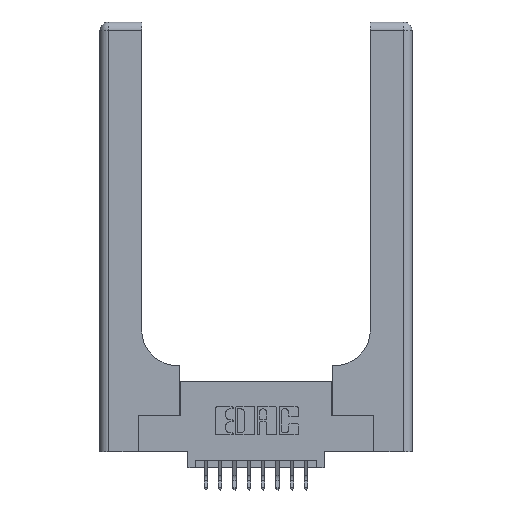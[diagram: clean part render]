
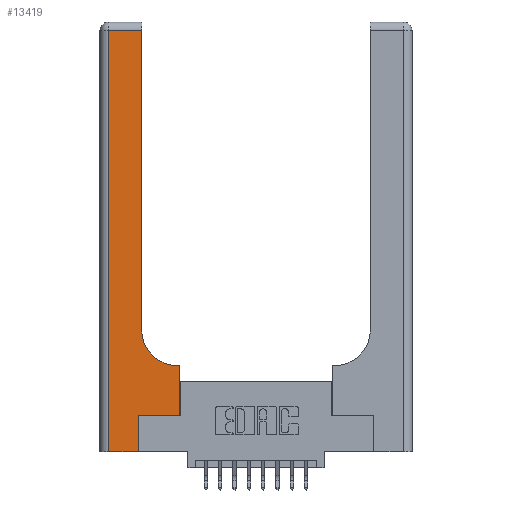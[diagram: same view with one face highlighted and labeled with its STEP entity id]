
A CAD part, top view. The second image highlights one B-rep face of the part: STEP entity #13419.
In plain terms, the highlighted planar face has unit normal (0, 0, 1).
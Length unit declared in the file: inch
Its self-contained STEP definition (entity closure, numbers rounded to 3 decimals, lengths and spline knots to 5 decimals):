
#223 = ORIENTED_EDGE ( 'NONE', *, *, #3497, .T. ) ;
#546 = CARTESIAN_POINT ( 'NONE',  ( 0., 0., 0.37 ) ) ;
#769 = CARTESIAN_POINT ( 'NONE',  ( 0.5585, 0.25, 0.37 ) ) ;
#796 = LINE ( 'NONE', #11181, #9317 ) ;
#807 = CARTESIAN_POINT ( 'NONE',  ( 0., 3., 0.37 ) ) ;
#1015 = EDGE_CURVE ( 'NONE', #10099, #3029, #2686, .T. ) ;
#1097 = VECTOR ( 'NONE', #10924, 39.37008 ) ;
#1381 = FACE_OUTER_BOUND ( 'NONE', #1650, .T. ) ;
#1394 = LINE ( 'NONE', #5864, #2605 ) ;
#1650 = EDGE_LOOP ( 'NONE', ( #8030, #5851, #15524, #223, #15790, #3409, #6822, #12961, #12147 ) ) ;
#1975 = DIRECTION ( 'NONE',  ( 1., 0., 0. ) ) ;
#1995 = VECTOR ( 'NONE', #3633, 39.37008 ) ;
#2091 = DIRECTION ( 'NONE',  ( -1., 0., 0. ) ) ;
#2115 = CARTESIAN_POINT ( 'NONE',  ( 0.269, 0., 0.37 ) ) ;
#2591 = CARTESIAN_POINT ( 'NONE',  ( 0.5415, 0.6, 0.37 ) ) ;
#2605 = VECTOR ( 'NONE', #5752, 39.37008 ) ;
#2686 = CIRCLE ( 'NONE', #16334, 0.25 ) ;
#3011 = CARTESIAN_POINT ( 'NONE',  ( 0.2915, 2.94, 0.37 ) ) ;
#3029 = VERTEX_POINT ( 'NONE', #15303 ) ;
#3409 = ORIENTED_EDGE ( 'NONE', *, *, #9844, .T. ) ;
#3497 = EDGE_CURVE ( 'NONE', #9450, #12011, #4415, .T. ) ;
#3633 = DIRECTION ( 'NONE',  ( 1., 0., 0. ) ) ;
#3676 = CARTESIAN_POINT ( 'NONE',  ( 0.06, 0., 0.37 ) ) ;
#4402 = DIRECTION ( 'NONE',  ( 0., 1., 0. ) ) ;
#4415 = LINE ( 'NONE', #546, #7609 ) ;
#4424 = EDGE_CURVE ( 'NONE', #12011, #5000, #15259, .T. ) ;
#4976 = EDGE_CURVE ( 'NONE', #3029, #5951, #13787, .T. ) ;
#5000 = VERTEX_POINT ( 'NONE', #8362 ) ;
#5591 = AXIS2_PLACEMENT_3D ( 'NONE', #807, #8357, #2091 ) ;
#5752 = DIRECTION ( 'NONE',  ( 0., -1., 0. ) ) ;
#5843 = DIRECTION ( 'NONE',  ( 0., 1., 0. ) ) ;
#5851 = ORIENTED_EDGE ( 'NONE', *, *, #7444, .T. ) ;
#5860 = LINE ( 'NONE', #7217, #11363 ) ;
#5864 = CARTESIAN_POINT ( 'NONE',  ( 0.06, 3., 0.37 ) ) ;
#5951 = VERTEX_POINT ( 'NONE', #3011 ) ;
#5972 = LINE ( 'NONE', #11192, #1995 ) ;
#5973 = CARTESIAN_POINT ( 'NONE',  ( 0., 2.94, 0.37 ) ) ;
#5976 = VECTOR ( 'NONE', #4402, 39.37008 ) ;
#6708 = CARTESIAN_POINT ( 'NONE',  ( 0.5585, 0.6, 0.37 ) ) ;
#6822 = ORIENTED_EDGE ( 'NONE', *, *, #12031, .T. ) ;
#6945 = CARTESIAN_POINT ( 'NONE',  ( 0.269, 0., 0.37 ) ) ;
#7028 = PLANE ( 'NONE',  #5591 ) ;
#7052 = VECTOR ( 'NONE', #5843, 39.37008 ) ;
#7217 = CARTESIAN_POINT ( 'NONE',  ( 0.5585, 0.25, 0.37 ) ) ;
#7444 = EDGE_CURVE ( 'NONE', #5951, #10582, #15350, .T. ) ;
#7609 = VECTOR ( 'NONE', #10572, 39.37008 ) ;
#8030 = ORIENTED_EDGE ( 'NONE', *, *, #4976, .T. ) ;
#8263 = VERTEX_POINT ( 'NONE', #769 ) ;
#8357 = DIRECTION ( 'NONE',  ( 0., 0., -1. ) ) ;
#8362 = CARTESIAN_POINT ( 'NONE',  ( 0.269, 0.25, 0.37 ) ) ;
#9317 = VECTOR ( 'NONE', #12285, 39.37008 ) ;
#9450 = VERTEX_POINT ( 'NONE', #3676 ) ;
#9515 = CARTESIAN_POINT ( 'NONE',  ( 0.2915, 3., 0.37 ) ) ;
#9567 = CARTESIAN_POINT ( 'NONE',  ( 0.5415, 0.85, 0.37 ) ) ;
#9844 = EDGE_CURVE ( 'NONE', #5000, #8263, #5972, .T. ) ;
#9939 = EDGE_CURVE ( 'NONE', #16413, #10099, #796, .T. ) ;
#10099 = VERTEX_POINT ( 'NONE', #2591 ) ;
#10572 = DIRECTION ( 'NONE',  ( 1., 0., 0. ) ) ;
#10582 = VERTEX_POINT ( 'NONE', #15832 ) ;
#10924 = DIRECTION ( 'NONE',  ( -1., 0., 0. ) ) ;
#11004 = DIRECTION ( 'NONE',  ( 0., 1., 0. ) ) ;
#11181 = CARTESIAN_POINT ( 'NONE',  ( 0.2915, 0.6, 0.37 ) ) ;
#11192 = CARTESIAN_POINT ( 'NONE',  ( 0.269, 0.25, 0.37 ) ) ;
#11363 = VECTOR ( 'NONE', #11004, 39.37008 ) ;
#12011 = VERTEX_POINT ( 'NONE', #2115 ) ;
#12031 = EDGE_CURVE ( 'NONE', #8263, #16413, #5860, .T. ) ;
#12147 = ORIENTED_EDGE ( 'NONE', *, *, #1015, .T. ) ;
#12285 = DIRECTION ( 'NONE',  ( -1., 0., 0. ) ) ;
#12961 = ORIENTED_EDGE ( 'NONE', *, *, #9939, .T. ) ;
#13021 = EDGE_CURVE ( 'NONE', #10582, #9450, #1394, .T. ) ;
#13419 = ADVANCED_FACE ( 'NONE', ( #1381 ), #7028, .F. ) ;
#13787 = LINE ( 'NONE', #9515, #7052 ) ;
#14656 = DIRECTION ( 'NONE',  ( 0., 0., -1. ) ) ;
#15259 = LINE ( 'NONE', #6945, #5976 ) ;
#15303 = CARTESIAN_POINT ( 'NONE',  ( 0.2915, 0.85, 0.37 ) ) ;
#15350 = LINE ( 'NONE', #5973, #1097 ) ;
#15524 = ORIENTED_EDGE ( 'NONE', *, *, #13021, .T. ) ;
#15790 = ORIENTED_EDGE ( 'NONE', *, *, #4424, .T. ) ;
#15832 = CARTESIAN_POINT ( 'NONE',  ( 0.06, 2.94, 0.37 ) ) ;
#16334 = AXIS2_PLACEMENT_3D ( 'NONE', #9567, #14656, #1975 ) ;
#16413 = VERTEX_POINT ( 'NONE', #6708 ) ;
